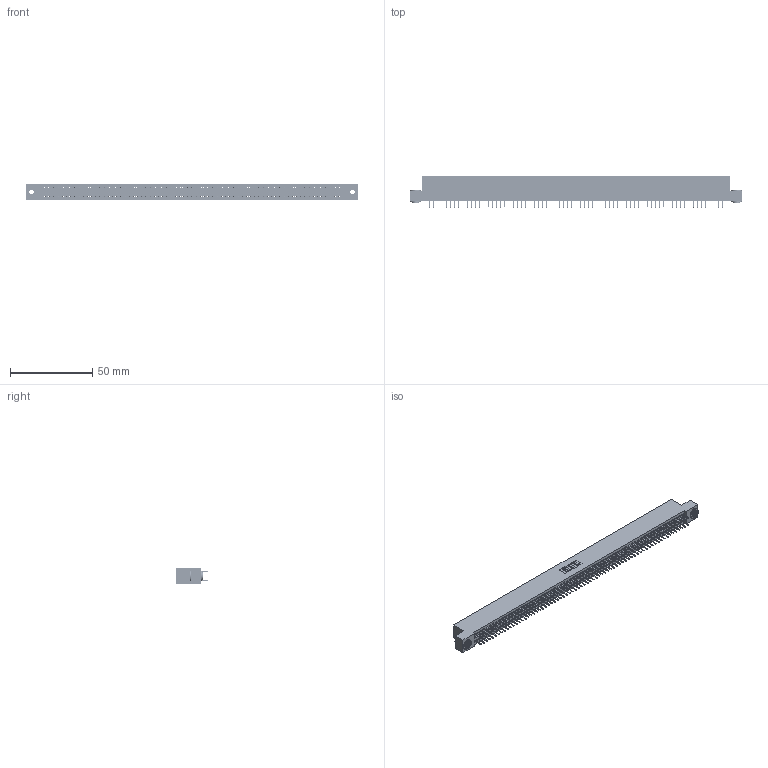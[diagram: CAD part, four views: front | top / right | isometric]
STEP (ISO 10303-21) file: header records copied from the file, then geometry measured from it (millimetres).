
FILE_DESCRIPTION (( 'STEP AP203' ), '1' );
FILE_NAME ('345-142-524-203.STEP', '2018-10-22T11:35:44', ( '' ), ( '' ), 'SwSTEP 2.0', 'SolidWorks 2016', '' );
FILE_SCHEMA (( 'CONFIG_CONTROL_DESIGN' ));
Length unit declared in the file: inch
Products named in the file (4): 345-292-001_345-293-124; 345-250-002_345-250-002-102; 345 Part_Flush Mounting Lugs - 0.156 Dia-TH; 345-142-524-203
Assembly tree (145 placements, depth 2):
  345-142-524-203
    345 Part_Flush Mounting Lugs - 0.156 Dia-TH
    345-292-001_345-293-124  x142
    345-250-002_345-250-002-102  x2
Bounding box: 201.55 x 19.35 x 9.4 mm (x, y, z)
Volume: 19652.4 mm3; surface area: 29248.8 mm2
Topology: 145 solids, 145 shells, 7832 faces, 22143 edges, 14190 vertices
Faces by surface type: plane 5628, cylinder 2196, cone 8
Entity records: 52528 total; most frequent: CARTESIAN_POINT 8751, ORIENTED_EDGE 8678, DIRECTION 7713, EDGE_CURVE 4339, LINE 3903, VECTOR 3903, VERTEX_POINT 2886, AXIS2_PLACEMENT_3D 1905
